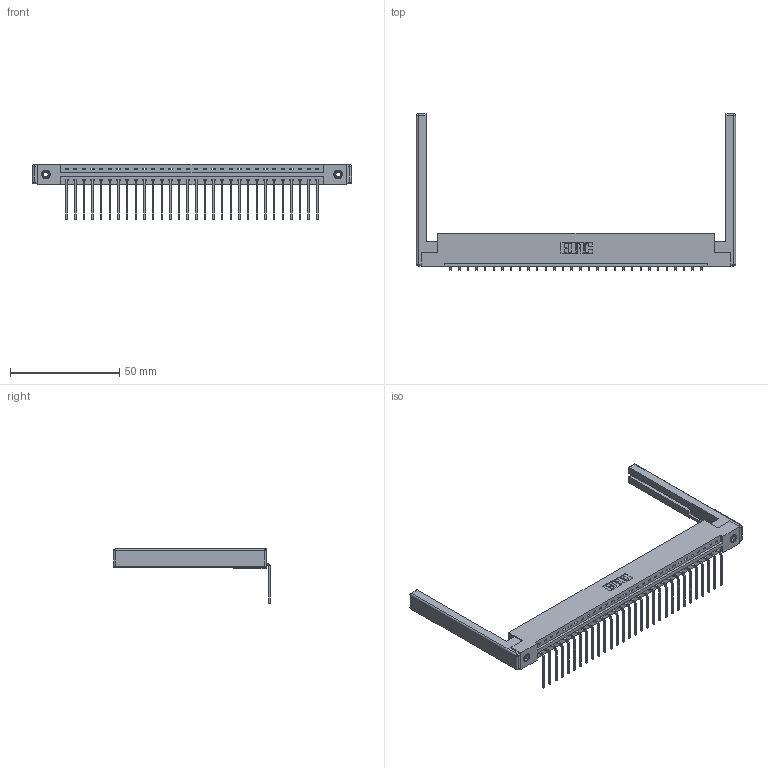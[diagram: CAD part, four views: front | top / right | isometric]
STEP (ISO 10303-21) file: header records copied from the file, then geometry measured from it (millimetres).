
FILE_DESCRIPTION (( 'STEP AP203' ), '1' );
FILE_NAME ('337-030-559-168.STEP', '2019-10-01T00:28:44', ( '' ), ( '' ), 'SwSTEP 2.0', 'SolidWorks 2016', '' );
FILE_SCHEMA (( 'CONFIG_CONTROL_DESIGN' ));
Length unit declared in the file: inch
Products named in the file (5): 337 Part_Flush Mounting Lugs - 0.156 Dia-TI; 307-220-068; 345-250-001_345-250-001-102; 337-030-559-168; 345-292-001_558 559 Tail - 1
Assembly tree (35 placements, depth 2):
  337-030-559-168
    337 Part_Flush Mounting Lugs - 0.156 Dia-TI
    345-292-001_558 559 Tail - 1  x30
    345-250-001_345-250-001-102  x2
    307-220-068  x2
Bounding box: 146.3 x 71.82 x 25.53 mm (x, y, z)
Volume: 19546.9 mm3; surface area: 20301.2 mm2
Topology: 35 solids, 35 shells, 2188 faces, 6521 edges, 4286 vertices
Faces by surface type: plane 1598, cylinder 566, cone 12, sphere 8, torus 4
Entity records: 26696 total; most frequent: CARTESIAN_POINT 4605, ORIENTED_EDGE 4560, DIRECTION 3974, EDGE_CURVE 2280, VECTOR 2102, LINE 2102, VERTEX_POINT 1510, AXIS2_PLACEMENT_3D 936
